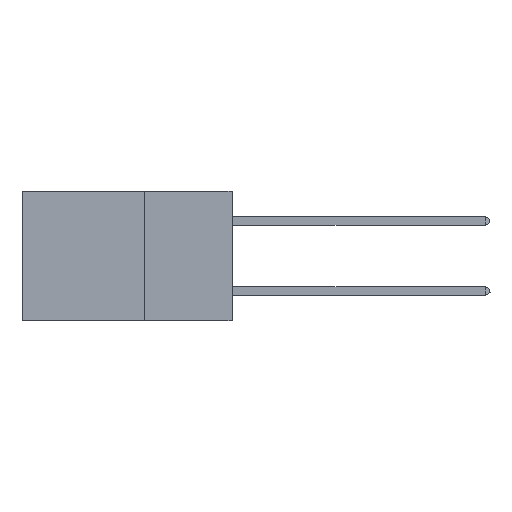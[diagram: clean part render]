
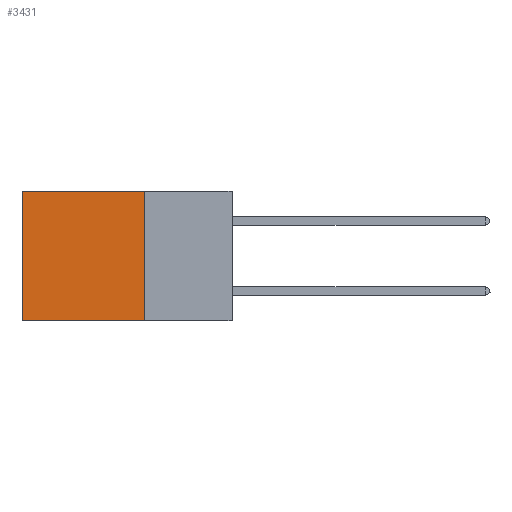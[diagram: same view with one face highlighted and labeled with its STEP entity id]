
A CAD part, left-side view. The second image highlights one B-rep face of the part: STEP entity #3431.
In plain terms, the highlighted planar face has unit normal (-1, 0, 0).
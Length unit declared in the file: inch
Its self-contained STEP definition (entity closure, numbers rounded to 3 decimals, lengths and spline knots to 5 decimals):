
#833 = CARTESIAN_POINT ( 'NONE',  ( 0.2875, 0.25, 0. ) ) ;
#852 = CARTESIAN_POINT ( 'NONE',  ( 0.2875, 0.6, 0. ) ) ;
#1033 = ORIENTED_EDGE ( 'NONE', *, *, #35339, .T. ) ;
#1650 = DIRECTION ( 'NONE',  ( 0., 0., -1. ) ) ;
#1652 = AXIS2_PLACEMENT_3D ( 'NONE', #38522, #42024, #21717 ) ;
#2188 = LINE ( 'NONE', #16191, #20388 ) ;
#3431 = ADVANCED_FACE ( 'NONE', ( #21510 ), #38672, .F. ) ;
#4082 = VECTOR ( 'NONE', #22202, 39.37008 ) ;
#5846 = LINE ( 'NONE', #8697, #41781 ) ;
#7546 = VERTEX_POINT ( 'NONE', #22889 ) ;
#8697 = CARTESIAN_POINT ( 'NONE',  ( 0.2875, 0.6, 0. ) ) ;
#10099 = DIRECTION ( 'NONE',  ( 0., 1., 0. ) ) ;
#11081 = EDGE_CURVE ( 'NONE', #23466, #26220, #2188, .T. ) ;
#13889 = LINE ( 'NONE', #42480, #4082 ) ;
#14014 = ORIENTED_EDGE ( 'NONE', *, *, #11081, .F. ) ;
#16191 = CARTESIAN_POINT ( 'NONE',  ( 0.2875, 0.25, 0. ) ) ;
#18493 = EDGE_LOOP ( 'NONE', ( #38355, #28079, #14014, #1033 ) ) ;
#19334 = EDGE_CURVE ( 'NONE', #26220, #7546, #13889, .T. ) ;
#20388 = VECTOR ( 'NONE', #1650, 39.37008 ) ;
#21480 = VERTEX_POINT ( 'NONE', #852 ) ;
#21510 = FACE_OUTER_BOUND ( 'NONE', #18493, .T. ) ;
#21717 = DIRECTION ( 'NONE',  ( 0., 0., -1. ) ) ;
#22202 = DIRECTION ( 'NONE',  ( 0., 1., 0. ) ) ;
#22889 = CARTESIAN_POINT ( 'NONE',  ( 0.2875, 0.6, -0.37 ) ) ;
#23466 = VERTEX_POINT ( 'NONE', #833 ) ;
#26220 = VERTEX_POINT ( 'NONE', #31544 ) ;
#26642 = VECTOR ( 'NONE', #10099, 39.37008 ) ;
#28079 = ORIENTED_EDGE ( 'NONE', *, *, #19334, .F. ) ;
#31145 = CARTESIAN_POINT ( 'NONE',  ( 0.2875, 0.25, 0. ) ) ;
#31544 = CARTESIAN_POINT ( 'NONE',  ( 0.2875, 0.25, -0.37 ) ) ;
#34610 = LINE ( 'NONE', #31145, #26642 ) ;
#35339 = EDGE_CURVE ( 'NONE', #23466, #21480, #34610, .T. ) ;
#36439 = EDGE_CURVE ( 'NONE', #21480, #7546, #5846, .T. ) ;
#36760 = DIRECTION ( 'NONE',  ( 0., 0., -1. ) ) ;
#38355 = ORIENTED_EDGE ( 'NONE', *, *, #36439, .T. ) ;
#38522 = CARTESIAN_POINT ( 'NONE',  ( 0.2875, 0.25, 0. ) ) ;
#38672 = PLANE ( 'NONE',  #1652 ) ;
#41781 = VECTOR ( 'NONE', #36760, 39.37008 ) ;
#42024 = DIRECTION ( 'NONE',  ( 1., 0., 0. ) ) ;
#42480 = CARTESIAN_POINT ( 'NONE',  ( 0.2875, 0.25, -0.37 ) ) ;
